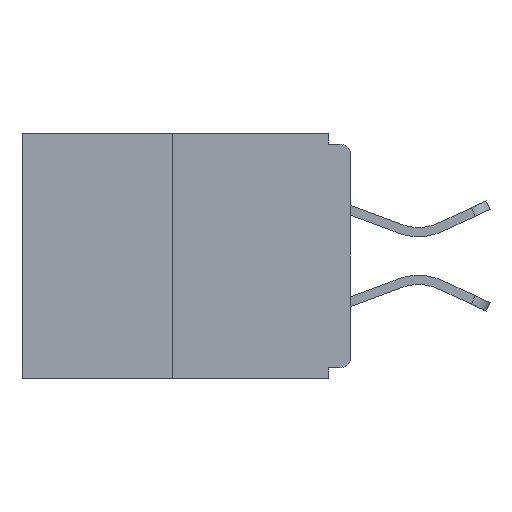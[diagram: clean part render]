
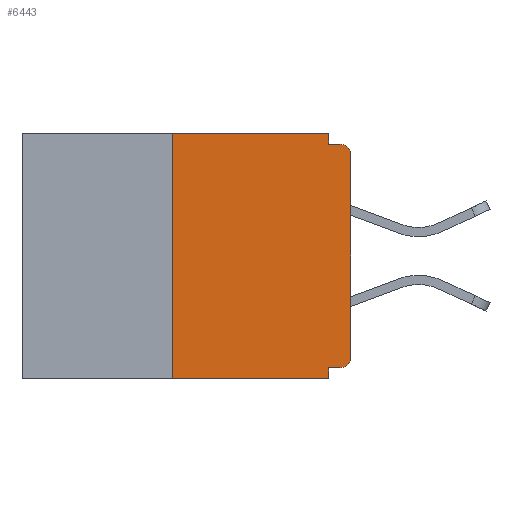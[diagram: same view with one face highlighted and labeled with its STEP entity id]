
A CAD part, left-side view. The second image highlights one B-rep face of the part: STEP entity #6443.
In plain terms, the highlighted planar face has unit normal (-1, 0, 0).
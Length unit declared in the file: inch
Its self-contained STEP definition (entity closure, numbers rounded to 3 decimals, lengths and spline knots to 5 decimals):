
#113 = DIRECTION ( 'NONE',  ( 1., 0., 0. ) ) ;
#144 = CARTESIAN_POINT ( 'NONE',  ( 0., 0., 0. ) ) ;
#176 = AXIS2_PLACEMENT_3D ( 'NONE', #5810, #113, #4670 ) ;
#190 = VERTEX_POINT ( 'NONE', #9463 ) ;
#207 = DIRECTION ( 'NONE',  ( -1., 0., 0. ) ) ;
#416 = DIRECTION ( 'NONE',  ( 0., 0., -1. ) ) ;
#810 = ORIENTED_EDGE ( 'NONE', *, *, #14970, .F. ) ;
#1140 = CARTESIAN_POINT ( 'NONE',  ( 0., 0.25, 0. ) ) ;
#1145 = VERTEX_POINT ( 'NONE', #4108 ) ;
#1295 = DIRECTION ( 'NONE',  ( 0., 0., 1. ) ) ;
#1299 = EDGE_CURVE ( 'NONE', #190, #12803, #14966, .T. ) ;
#1496 = LINE ( 'NONE', #9859, #14126 ) ;
#1514 = VECTOR ( 'NONE', #8412, 39.37008 ) ;
#1707 = CARTESIAN_POINT ( 'NONE',  ( 0., 0.031, -0.328 ) ) ;
#2008 = DIRECTION ( 'NONE',  ( -1., 0., 0. ) ) ;
#2041 = LINE ( 'NONE', #10720, #3508 ) ;
#2445 = ORIENTED_EDGE ( 'NONE', *, *, #13556, .F. ) ;
#2493 = ORIENTED_EDGE ( 'NONE', *, *, #3295, .T. ) ;
#2541 = VERTEX_POINT ( 'NONE', #5828 ) ;
#2616 = VECTOR ( 'NONE', #6033, 39.37008 ) ;
#2689 = LINE ( 'NONE', #5219, #3637 ) ;
#2959 = CARTESIAN_POINT ( 'NONE',  ( 0., 0., -0.03 ) ) ;
#3295 = EDGE_CURVE ( 'NONE', #10763, #14090, #14147, .T. ) ;
#3508 = VECTOR ( 'NONE', #12003, 39.37008 ) ;
#3528 = CARTESIAN_POINT ( 'NONE',  ( 0., 0.46, 0. ) ) ;
#3637 = VECTOR ( 'NONE', #11100, 39.37008 ) ;
#4108 = CARTESIAN_POINT ( 'NONE',  ( 0., 0.031, -0.343 ) ) ;
#4513 = CARTESIAN_POINT ( 'NONE',  ( 0., 0.031, -0.015 ) ) ;
#4670 = DIRECTION ( 'NONE',  ( 0., 0., -1. ) ) ;
#5211 = ORIENTED_EDGE ( 'NONE', *, *, #11454, .T. ) ;
#5219 = CARTESIAN_POINT ( 'NONE',  ( 0., 0., -0.015 ) ) ;
#5411 = VERTEX_POINT ( 'NONE', #4513 ) ;
#5510 = ORIENTED_EDGE ( 'NONE', *, *, #15327, .F. ) ;
#5810 = CARTESIAN_POINT ( 'NONE',  ( 0., 0.46, 0. ) ) ;
#5828 = CARTESIAN_POINT ( 'NONE',  ( 0., 0.25, -0.343 ) ) ;
#6033 = DIRECTION ( 'NONE',  ( 0., 1., 0. ) ) ;
#6443 = ADVANCED_FACE ( 'NONE', ( #12987 ), #15306, .F. ) ;
#6505 = EDGE_CURVE ( 'NONE', #2541, #190, #13173, .T. ) ;
#6701 = CARTESIAN_POINT ( 'NONE',  ( 0., 0.015, -0.03 ) ) ;
#7299 = CIRCLE ( 'NONE', #8733, 0.015 ) ;
#8169 = VERTEX_POINT ( 'NONE', #1707 ) ;
#8272 = CARTESIAN_POINT ( 'NONE',  ( 0., 0., -0.328 ) ) ;
#8359 = VERTEX_POINT ( 'NONE', #13234 ) ;
#8412 = DIRECTION ( 'NONE',  ( 0., 0., 1. ) ) ;
#8733 = AXIS2_PLACEMENT_3D ( 'NONE', #6701, #2008, #14951 ) ;
#8982 = ORIENTED_EDGE ( 'NONE', *, *, #6505, .F. ) ;
#9052 = VECTOR ( 'NONE', #10430, 39.37008 ) ;
#9463 = CARTESIAN_POINT ( 'NONE',  ( 0., 0.25, 0. ) ) ;
#9647 = DIRECTION ( 'NONE',  ( 0., -1., 0. ) ) ;
#9859 = CARTESIAN_POINT ( 'NONE',  ( 0., 0.46, -0.343 ) ) ;
#10061 = AXIS2_PLACEMENT_3D ( 'NONE', #13286, #207, #416 ) ;
#10430 = DIRECTION ( 'NONE',  ( 0., 0., -1. ) ) ;
#10504 = EDGE_CURVE ( 'NONE', #2541, #1145, #1496, .T. ) ;
#10632 = CARTESIAN_POINT ( 'NONE',  ( 0., 0., -0.313 ) ) ;
#10637 = LINE ( 'NONE', #8272, #2616 ) ;
#10668 = VERTEX_POINT ( 'NONE', #15238 ) ;
#10720 = CARTESIAN_POINT ( 'NONE',  ( 0., 0.031, 0. ) ) ;
#10763 = VERTEX_POINT ( 'NONE', #10632 ) ;
#10899 = EDGE_CURVE ( 'NONE', #10668, #10763, #10904, .T. ) ;
#10904 = CIRCLE ( 'NONE', #10061, 0.015 ) ;
#11100 = DIRECTION ( 'NONE',  ( 0., -1., 0. ) ) ;
#11224 = EDGE_LOOP ( 'NONE', ( #14557, #8982, #12972, #810, #12334, #14058, #2493, #5211, #5510, #2445 ) ) ;
#11454 = EDGE_CURVE ( 'NONE', #14090, #8359, #7299, .T. ) ;
#11557 = CARTESIAN_POINT ( 'NONE',  ( 0., 0.031, -0.343 ) ) ;
#12003 = DIRECTION ( 'NONE',  ( 0., 0., -1. ) ) ;
#12334 = ORIENTED_EDGE ( 'NONE', *, *, #12489, .F. ) ;
#12489 = EDGE_CURVE ( 'NONE', #10668, #8169, #10637, .T. ) ;
#12803 = VERTEX_POINT ( 'NONE', #12817 ) ;
#12817 = CARTESIAN_POINT ( 'NONE',  ( 0., 0.031, 0. ) ) ;
#12972 = ORIENTED_EDGE ( 'NONE', *, *, #10504, .T. ) ;
#12987 = FACE_OUTER_BOUND ( 'NONE', #11224, .T. ) ;
#13173 = LINE ( 'NONE', #1140, #15015 ) ;
#13234 = CARTESIAN_POINT ( 'NONE',  ( 0., 0.015, -0.015 ) ) ;
#13286 = CARTESIAN_POINT ( 'NONE',  ( 0., 0.015, -0.313 ) ) ;
#13556 = EDGE_CURVE ( 'NONE', #12803, #5411, #2041, .T. ) ;
#13847 = VECTOR ( 'NONE', #14261, 39.37008 ) ;
#14058 = ORIENTED_EDGE ( 'NONE', *, *, #10899, .T. ) ;
#14090 = VERTEX_POINT ( 'NONE', #2959 ) ;
#14126 = VECTOR ( 'NONE', #9647, 39.37008 ) ;
#14147 = LINE ( 'NONE', #144, #1514 ) ;
#14261 = DIRECTION ( 'NONE',  ( 0., -1., 0. ) ) ;
#14268 = LINE ( 'NONE', #11557, #9052 ) ;
#14557 = ORIENTED_EDGE ( 'NONE', *, *, #1299, .F. ) ;
#14951 = DIRECTION ( 'NONE',  ( 0., 0., -1. ) ) ;
#14966 = LINE ( 'NONE', #3528, #13847 ) ;
#14970 = EDGE_CURVE ( 'NONE', #8169, #1145, #14268, .T. ) ;
#15015 = VECTOR ( 'NONE', #1295, 39.37008 ) ;
#15238 = CARTESIAN_POINT ( 'NONE',  ( 0., 0.015, -0.328 ) ) ;
#15306 = PLANE ( 'NONE',  #176 ) ;
#15327 = EDGE_CURVE ( 'NONE', #5411, #8359, #2689, .T. ) ;
